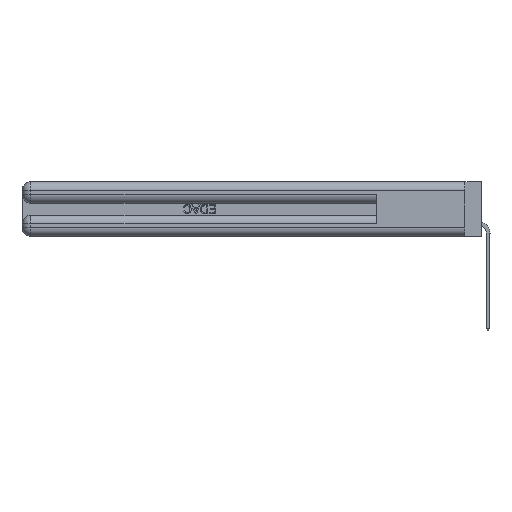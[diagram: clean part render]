
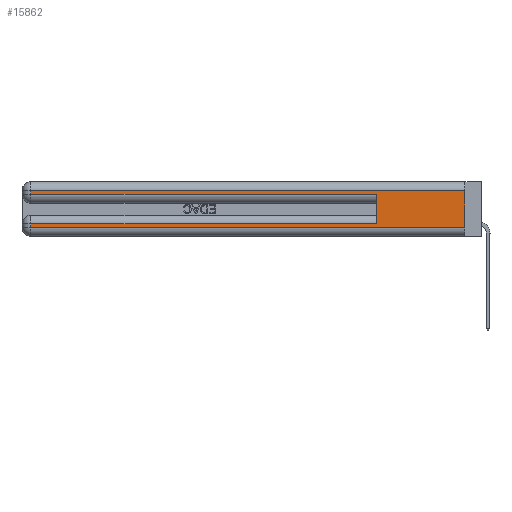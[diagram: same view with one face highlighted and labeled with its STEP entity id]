
A CAD part, left-side view. The second image highlights one B-rep face of the part: STEP entity #15862.
In plain terms, the highlighted planar face has unit normal (-1, 0, 0).
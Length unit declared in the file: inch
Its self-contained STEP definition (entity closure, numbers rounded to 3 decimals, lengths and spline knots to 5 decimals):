
#1107 = LINE ( 'NONE', #23118, #34495 ) ;
#2108 = AXIS2_PLACEMENT_3D ( 'NONE', #31210, #19037, #21873 ) ;
#2214 = PLANE ( 'NONE',  #2108 ) ;
#2773 = ORIENTED_EDGE ( 'NONE', *, *, #23131, .F. ) ;
#3438 = VERTEX_POINT ( 'NONE', #20749 ) ;
#3914 = LINE ( 'NONE', #10697, #13604 ) ;
#4042 = VERTEX_POINT ( 'NONE', #10621 ) ;
#4106 = DIRECTION ( 'NONE',  ( 0., 0., -1. ) ) ;
#5101 = CARTESIAN_POINT ( 'NONE',  ( 0., 2.94, 0.37 ) ) ;
#5262 = CARTESIAN_POINT ( 'NONE',  ( 0., 0.6, 0.145 ) ) ;
#5293 = VECTOR ( 'NONE', #19881, 39.37008 ) ;
#5892 = EDGE_CURVE ( 'NONE', #30280, #19791, #18234, .T. ) ;
#6853 = VECTOR ( 'NONE', #7719, 39.37008 ) ;
#7351 = ORIENTED_EDGE ( 'NONE', *, *, #28567, .T. ) ;
#7535 = LINE ( 'NONE', #5101, #14123 ) ;
#7719 = DIRECTION ( 'NONE',  ( 0., 0., 1. ) ) ;
#8757 = EDGE_LOOP ( 'NONE', ( #12901, #14496, #34800, #30435, #2773, #23734, #7351, #25086 ) ) ;
#10288 = DIRECTION ( 'NONE',  ( 0., 0., -1. ) ) ;
#10613 = CARTESIAN_POINT ( 'NONE',  ( 0., 0.6, 0.085 ) ) ;
#10621 = CARTESIAN_POINT ( 'NONE',  ( 0., 2.94, 0.085 ) ) ;
#10697 = CARTESIAN_POINT ( 'NONE',  ( 0., 0., 0.06 ) ) ;
#11456 = CARTESIAN_POINT ( 'NONE',  ( 0., 2.94, 0.285 ) ) ;
#12901 = ORIENTED_EDGE ( 'NONE', *, *, #28606, .F. ) ;
#13457 = CARTESIAN_POINT ( 'NONE',  ( 0., 0., 0.06 ) ) ;
#13604 = VECTOR ( 'NONE', #36197, 39.37008 ) ;
#14123 = VECTOR ( 'NONE', #10288, 39.37008 ) ;
#14341 = LINE ( 'NONE', #5262, #6853 ) ;
#14496 = ORIENTED_EDGE ( 'NONE', *, *, #5892, .T. ) ;
#15862 = ADVANCED_FACE ( 'NONE', ( #22649 ), #2214, .F. ) ;
#16441 = EDGE_CURVE ( 'NONE', #18421, #4042, #1107, .T. ) ;
#18234 = LINE ( 'NONE', #32403, #28349 ) ;
#18375 = DIRECTION ( 'NONE',  ( 0., 1., 0. ) ) ;
#18421 = VERTEX_POINT ( 'NONE', #10613 ) ;
#18745 = VECTOR ( 'NONE', #4106, 39.37008 ) ;
#19037 = DIRECTION ( 'NONE',  ( 1., 0., 0. ) ) ;
#19583 = DIRECTION ( 'NONE',  ( 0., 0., -1. ) ) ;
#19791 = VERTEX_POINT ( 'NONE', #29519 ) ;
#19881 = DIRECTION ( 'NONE',  ( 0., -1., 0. ) ) ;
#20053 = VERTEX_POINT ( 'NONE', #11456 ) ;
#20749 = CARTESIAN_POINT ( 'NONE',  ( 0., 0.6, 0.285 ) ) ;
#20857 = EDGE_CURVE ( 'NONE', #20053, #3438, #35577, .T. ) ;
#21383 = EDGE_CURVE ( 'NONE', #27591, #28589, #3914, .T. ) ;
#21873 = DIRECTION ( 'NONE',  ( 0., 0., -1. ) ) ;
#22533 = CARTESIAN_POINT ( 'NONE',  ( 0., 0., 0.37 ) ) ;
#22615 = CARTESIAN_POINT ( 'NONE',  ( 0., 2.94, 0.06 ) ) ;
#22649 = FACE_OUTER_BOUND ( 'NONE', #8757, .T. ) ;
#22883 = VECTOR ( 'NONE', #19583, 39.37008 ) ;
#23118 = CARTESIAN_POINT ( 'NONE',  ( 0., 0., 0.085 ) ) ;
#23131 = EDGE_CURVE ( 'NONE', #18421, #3438, #14341, .T. ) ;
#23734 = ORIENTED_EDGE ( 'NONE', *, *, #16441, .T. ) ;
#23771 = EDGE_CURVE ( 'NONE', #19791, #20053, #34542, .T. ) ;
#25086 = ORIENTED_EDGE ( 'NONE', *, *, #21383, .T. ) ;
#26458 = CARTESIAN_POINT ( 'NONE',  ( 0., 2.94, 0.37 ) ) ;
#26828 = LINE ( 'NONE', #22533, #22883 ) ;
#27591 = VERTEX_POINT ( 'NONE', #22615 ) ;
#28349 = VECTOR ( 'NONE', #18375, 39.37008 ) ;
#28567 = EDGE_CURVE ( 'NONE', #4042, #27591, #7535, .T. ) ;
#28589 = VERTEX_POINT ( 'NONE', #13457 ) ;
#28606 = EDGE_CURVE ( 'NONE', #30280, #28589, #26828, .T. ) ;
#29519 = CARTESIAN_POINT ( 'NONE',  ( 0., 2.94, 0.31 ) ) ;
#30280 = VERTEX_POINT ( 'NONE', #33887 ) ;
#30435 = ORIENTED_EDGE ( 'NONE', *, *, #20857, .T. ) ;
#30599 = CARTESIAN_POINT ( 'NONE',  ( 0., 0., 0.285 ) ) ;
#31210 = CARTESIAN_POINT ( 'NONE',  ( 0., 0., 0.37 ) ) ;
#32403 = CARTESIAN_POINT ( 'NONE',  ( 0., 0., 0.31 ) ) ;
#33887 = CARTESIAN_POINT ( 'NONE',  ( 0., 0., 0.31 ) ) ;
#34063 = DIRECTION ( 'NONE',  ( 0., 1., 0. ) ) ;
#34495 = VECTOR ( 'NONE', #34063, 39.37008 ) ;
#34542 = LINE ( 'NONE', #26458, #18745 ) ;
#34800 = ORIENTED_EDGE ( 'NONE', *, *, #23771, .T. ) ;
#35577 = LINE ( 'NONE', #30599, #5293 ) ;
#36197 = DIRECTION ( 'NONE',  ( 0., -1., 0. ) ) ;
